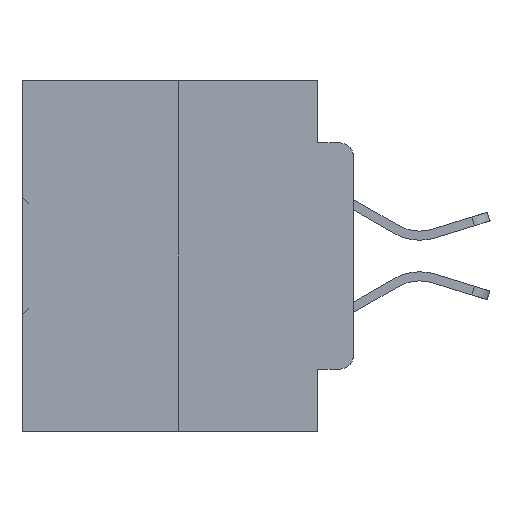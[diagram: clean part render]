
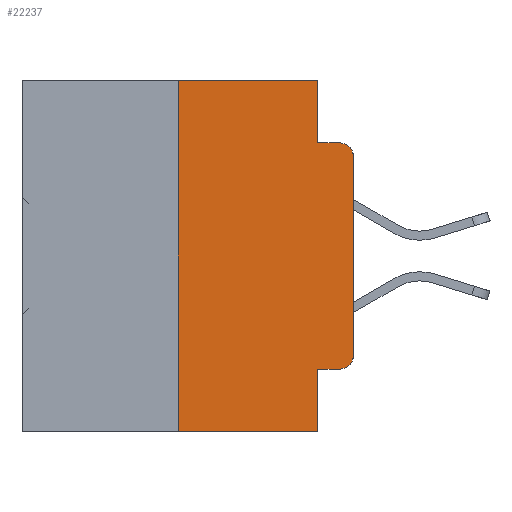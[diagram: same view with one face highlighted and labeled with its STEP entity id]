
A CAD part, left-side view. The second image highlights one B-rep face of the part: STEP entity #22237.
In plain terms, the highlighted planar face has unit normal (-1, 0, 0).
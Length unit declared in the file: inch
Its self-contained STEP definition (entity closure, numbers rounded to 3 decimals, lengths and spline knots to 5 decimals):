
#672 = DIRECTION ( 'NONE',  ( 0., -1., 0. ) ) ;
#1202 = LINE ( 'NONE', #28797, #16355 ) ;
#2067 = EDGE_CURVE ( 'NONE', #22757, #8076, #36749, .T. ) ;
#2164 = CARTESIAN_POINT ( 'NONE',  ( 0., 0.051, -0.4115 ) ) ;
#2450 = VECTOR ( 'NONE', #672, 39.37008 ) ;
#2616 = VERTEX_POINT ( 'NONE', #29687 ) ;
#3547 = EDGE_CURVE ( 'NONE', #37825, #22757, #26129, .T. ) ;
#4030 = ORIENTED_EDGE ( 'NONE', *, *, #19410, .T. ) ;
#4191 = CIRCLE ( 'NONE', #14746, 0.02 ) ;
#5373 = DIRECTION ( 'NONE',  ( 0., 0., 1. ) ) ;
#5506 = CARTESIAN_POINT ( 'NONE',  ( 0., 0.051, 0. ) ) ;
#5696 = EDGE_CURVE ( 'NONE', #31301, #37825, #22805, .T. ) ;
#7027 = EDGE_CURVE ( 'NONE', #12771, #2616, #17570, .T. ) ;
#7097 = CARTESIAN_POINT ( 'NONE',  ( 0., 0.02, -0.1085 ) ) ;
#7227 = VECTOR ( 'NONE', #25183, 39.37008 ) ;
#7327 = CARTESIAN_POINT ( 'NONE',  ( 0., 0.02, -0.3915 ) ) ;
#7950 = CARTESIAN_POINT ( 'NONE',  ( 0., 0.25, -0.5 ) ) ;
#8076 = VERTEX_POINT ( 'NONE', #36996 ) ;
#8721 = DIRECTION ( 'NONE',  ( 0., 0., -1. ) ) ;
#9064 = ORIENTED_EDGE ( 'NONE', *, *, #30399, .T. ) ;
#10028 = VECTOR ( 'NONE', #20808, 39.37008 ) ;
#10069 = EDGE_CURVE ( 'NONE', #15849, #19055, #16939, .T. ) ;
#10484 = EDGE_CURVE ( 'NONE', #12771, #30229, #30139, .T. ) ;
#12143 = LINE ( 'NONE', #19528, #24483 ) ;
#12771 = VERTEX_POINT ( 'NONE', #32092 ) ;
#14375 = EDGE_CURVE ( 'NONE', #19055, #8076, #4191, .T. ) ;
#14481 = DIRECTION ( 'NONE',  ( 1., 0., 0. ) ) ;
#14746 = AXIS2_PLACEMENT_3D ( 'NONE', #7097, #27565, #30507 ) ;
#15118 = CARTESIAN_POINT ( 'NONE',  ( 0., 0.051, 0. ) ) ;
#15365 = VERTEX_POINT ( 'NONE', #7950 ) ;
#15849 = VERTEX_POINT ( 'NONE', #27956 ) ;
#16355 = VECTOR ( 'NONE', #5373, 39.37008 ) ;
#16939 = LINE ( 'NONE', #17556, #10028 ) ;
#17036 = ORIENTED_EDGE ( 'NONE', *, *, #2067, .F. ) ;
#17485 = CARTESIAN_POINT ( 'NONE',  ( 0., 0.25, 0. ) ) ;
#17556 = CARTESIAN_POINT ( 'NONE',  ( 0., 0., 0. ) ) ;
#17570 = LINE ( 'NONE', #19137, #28534 ) ;
#18061 = ORIENTED_EDGE ( 'NONE', *, *, #10484, .T. ) ;
#18080 = ORIENTED_EDGE ( 'NONE', *, *, #10069, .T. ) ;
#18385 = AXIS2_PLACEMENT_3D ( 'NONE', #34410, #14481, #34928 ) ;
#18827 = DIRECTION ( 'NONE',  ( -1., 0., 0. ) ) ;
#19055 = VERTEX_POINT ( 'NONE', #32713 ) ;
#19137 = CARTESIAN_POINT ( 'NONE',  ( 0., 0.051, 0. ) ) ;
#19410 = EDGE_CURVE ( 'NONE', #30229, #15849, #31405, .T. ) ;
#19528 = CARTESIAN_POINT ( 'NONE',  ( 0., 0.473, -0.5 ) ) ;
#20808 = DIRECTION ( 'NONE',  ( 0., 0., 1. ) ) ;
#22237 = ADVANCED_FACE ( 'NONE', ( #24316 ), #31586, .F. ) ;
#22757 = VERTEX_POINT ( 'NONE', #23833 ) ;
#22805 = LINE ( 'NONE', #26389, #31508 ) ;
#22874 = ORIENTED_EDGE ( 'NONE', *, *, #3547, .F. ) ;
#23833 = CARTESIAN_POINT ( 'NONE',  ( 0., 0.051, -0.0885 ) ) ;
#24316 = FACE_OUTER_BOUND ( 'NONE', #29578, .T. ) ;
#24483 = VECTOR ( 'NONE', #30909, 39.37008 ) ;
#24776 = DIRECTION ( 'NONE',  ( 0., 0., -1. ) ) ;
#24784 = ORIENTED_EDGE ( 'NONE', *, *, #14375, .T. ) ;
#25183 = DIRECTION ( 'NONE',  ( 0., -1., 0. ) ) ;
#26129 = LINE ( 'NONE', #5506, #27493 ) ;
#26148 = DIRECTION ( 'NONE',  ( 0., -1., 0. ) ) ;
#26389 = CARTESIAN_POINT ( 'NONE',  ( 0., 0.473, 0. ) ) ;
#27493 = VECTOR ( 'NONE', #8721, 39.37008 ) ;
#27565 = DIRECTION ( 'NONE',  ( -1., 0., 0. ) ) ;
#27956 = CARTESIAN_POINT ( 'NONE',  ( 0., 0., -0.3915 ) ) ;
#28534 = VECTOR ( 'NONE', #24776, 39.37008 ) ;
#28797 = CARTESIAN_POINT ( 'NONE',  ( 0., 0.25, 0. ) ) ;
#29111 = ORIENTED_EDGE ( 'NONE', *, *, #5696, .F. ) ;
#29578 = EDGE_LOOP ( 'NONE', ( #18080, #24784, #17036, #22874, #29111, #36662, #9064, #33821, #18061, #4030 ) ) ;
#29687 = CARTESIAN_POINT ( 'NONE',  ( 0., 0.051, -0.5 ) ) ;
#29957 = EDGE_CURVE ( 'NONE', #15365, #31301, #1202, .T. ) ;
#30139 = LINE ( 'NONE', #2164, #7227 ) ;
#30229 = VERTEX_POINT ( 'NONE', #35790 ) ;
#30399 = EDGE_CURVE ( 'NONE', #15365, #2616, #12143, .T. ) ;
#30507 = DIRECTION ( 'NONE',  ( 0., 0., -1. ) ) ;
#30909 = DIRECTION ( 'NONE',  ( 0., -1., 0. ) ) ;
#31301 = VERTEX_POINT ( 'NONE', #17485 ) ;
#31405 = CIRCLE ( 'NONE', #34461, 0.02 ) ;
#31508 = VECTOR ( 'NONE', #26148, 39.37008 ) ;
#31586 = PLANE ( 'NONE',  #18385 ) ;
#32092 = CARTESIAN_POINT ( 'NONE',  ( 0., 0.051, -0.4115 ) ) ;
#32713 = CARTESIAN_POINT ( 'NONE',  ( 0., 0., -0.1085 ) ) ;
#33821 = ORIENTED_EDGE ( 'NONE', *, *, #7027, .F. ) ;
#34410 = CARTESIAN_POINT ( 'NONE',  ( 0., 0.473, 0. ) ) ;
#34461 = AXIS2_PLACEMENT_3D ( 'NONE', #7327, #18827, #36624 ) ;
#34928 = DIRECTION ( 'NONE',  ( 0., 0., -1. ) ) ;
#35225 = CARTESIAN_POINT ( 'NONE',  ( 0., 0.051, -0.0885 ) ) ;
#35790 = CARTESIAN_POINT ( 'NONE',  ( 0., 0.02, -0.4115 ) ) ;
#36624 = DIRECTION ( 'NONE',  ( 0., 0., -1. ) ) ;
#36662 = ORIENTED_EDGE ( 'NONE', *, *, #29957, .F. ) ;
#36749 = LINE ( 'NONE', #35225, #2450 ) ;
#36996 = CARTESIAN_POINT ( 'NONE',  ( 0., 0.02, -0.0885 ) ) ;
#37825 = VERTEX_POINT ( 'NONE', #15118 ) ;
